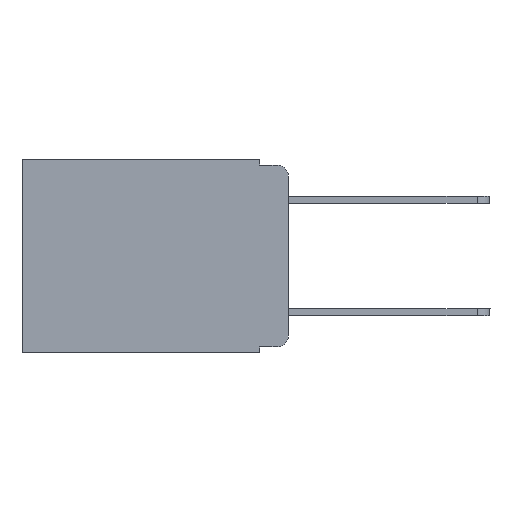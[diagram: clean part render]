
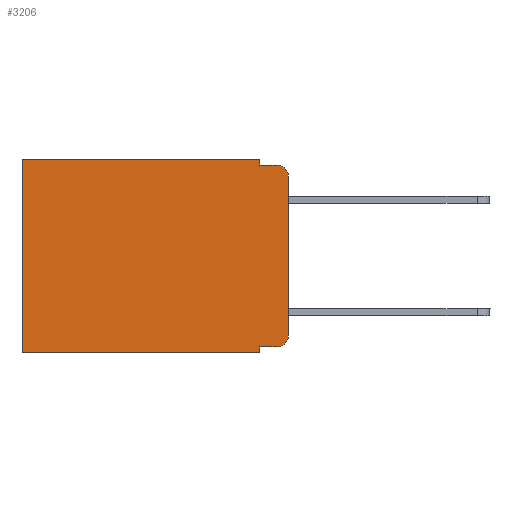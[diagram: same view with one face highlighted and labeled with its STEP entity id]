
A CAD part, left-side view. The second image highlights one B-rep face of the part: STEP entity #3206.
In plain terms, the highlighted planar face has unit normal (-1, 0, 0).
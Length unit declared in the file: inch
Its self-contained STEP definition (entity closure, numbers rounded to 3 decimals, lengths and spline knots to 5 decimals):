
#58 = DIRECTION ( 'NONE',  ( 1., 0., 0. ) ) ;
#177 = VERTEX_POINT ( 'NONE', #828 ) ;
#245 = VECTOR ( 'NONE', #8202, 39.37008 ) ;
#268 = CARTESIAN_POINT ( 'NONE',  ( 0.298, 0.051, -0.01 ) ) ;
#376 = VECTOR ( 'NONE', #6750, 39.37008 ) ;
#405 = VERTEX_POINT ( 'NONE', #2951 ) ;
#440 = EDGE_CURVE ( 'NONE', #177, #8833, #8044, .T. ) ;
#578 = ORIENTED_EDGE ( 'NONE', *, *, #5057, .T. ) ;
#694 = LINE ( 'NONE', #5782, #376 ) ;
#828 = CARTESIAN_POINT ( 'NONE',  ( 0.298, 0., -0.03 ) ) ;
#848 = AXIS2_PLACEMENT_3D ( 'NONE', #11522, #58, #8780 ) ;
#969 = EDGE_CURVE ( 'NONE', #11356, #11102, #1796, .T. ) ;
#1098 = CARTESIAN_POINT ( 'NONE',  ( 0.298, 0.473, 0. ) ) ;
#1139 = CARTESIAN_POINT ( 'NONE',  ( 0.298, 0., 0. ) ) ;
#1166 = DIRECTION ( 'NONE',  ( 0., -1., 0. ) ) ;
#1343 = VECTOR ( 'NONE', #5921, 39.37008 ) ;
#1364 = CARTESIAN_POINT ( 'NONE',  ( 0.298, 0.051, 0. ) ) ;
#1660 = EDGE_CURVE ( 'NONE', #2913, #10667, #4234, .T. ) ;
#1796 = LINE ( 'NONE', #1139, #1343 ) ;
#2114 = ORIENTED_EDGE ( 'NONE', *, *, #2936, .F. ) ;
#2369 = ORIENTED_EDGE ( 'NONE', *, *, #4551, .F. ) ;
#2622 = LINE ( 'NONE', #268, #12296 ) ;
#2631 = VERTEX_POINT ( 'NONE', #12217 ) ;
#2913 = VERTEX_POINT ( 'NONE', #6531 ) ;
#2936 = EDGE_CURVE ( 'NONE', #6580, #405, #11005, .T. ) ;
#2951 = CARTESIAN_POINT ( 'NONE',  ( 0.298, 0.473, -0.343 ) ) ;
#2954 = ORIENTED_EDGE ( 'NONE', *, *, #4802, .F. ) ;
#3108 = ORIENTED_EDGE ( 'NONE', *, *, #440, .T. ) ;
#3206 = ADVANCED_FACE ( 'NONE', ( #6634 ), #10573, .F. ) ;
#3431 = DIRECTION ( 'NONE',  ( 0., -1., 0. ) ) ;
#3469 = CARTESIAN_POINT ( 'NONE',  ( 0.298, 0., -0.343 ) ) ;
#3478 = CARTESIAN_POINT ( 'NONE',  ( 0.298, 0.02, -0.333 ) ) ;
#3560 = CARTESIAN_POINT ( 'NONE',  ( 0.298, 0.051, -0.333 ) ) ;
#3712 = EDGE_CURVE ( 'NONE', #11356, #5289, #694, .T. ) ;
#3851 = CARTESIAN_POINT ( 'NONE',  ( 0.298, 0.02, -0.313 ) ) ;
#4076 = ORIENTED_EDGE ( 'NONE', *, *, #969, .T. ) ;
#4234 = LINE ( 'NONE', #3560, #6826 ) ;
#4291 = DIRECTION ( 'NONE',  ( 0., 0., -1. ) ) ;
#4551 = EDGE_CURVE ( 'NONE', #177, #2631, #7924, .T. ) ;
#4648 = CIRCLE ( 'NONE', #8745, 0.02 ) ;
#4802 = EDGE_CURVE ( 'NONE', #5289, #8833, #2622, .T. ) ;
#5057 = EDGE_CURVE ( 'NONE', #11102, #405, #11379, .T. ) ;
#5289 = VERTEX_POINT ( 'NONE', #10189 ) ;
#5382 = DIRECTION ( 'NONE',  ( -1., 0., 0. ) ) ;
#5421 = CARTESIAN_POINT ( 'NONE',  ( 0.298, 0.02, -0.03 ) ) ;
#5782 = CARTESIAN_POINT ( 'NONE',  ( 0.298, 0.051, 0. ) ) ;
#5921 = DIRECTION ( 'NONE',  ( 0., 1., 0. ) ) ;
#6219 = CARTESIAN_POINT ( 'NONE',  ( 0.298, 0., 0. ) ) ;
#6531 = CARTESIAN_POINT ( 'NONE',  ( 0.298, 0.051, -0.333 ) ) ;
#6580 = VERTEX_POINT ( 'NONE', #11463 ) ;
#6634 = FACE_OUTER_BOUND ( 'NONE', #9726, .T. ) ;
#6750 = DIRECTION ( 'NONE',  ( 0., 0., -1. ) ) ;
#6792 = DIRECTION ( 'NONE',  ( 0., 0., -1. ) ) ;
#6826 = VECTOR ( 'NONE', #3431, 39.37008 ) ;
#7299 = CARTESIAN_POINT ( 'NONE',  ( 0.298, 0.02, -0.01 ) ) ;
#7401 = VECTOR ( 'NONE', #10286, 39.37008 ) ;
#7889 = DIRECTION ( 'NONE',  ( 0., 0., -1. ) ) ;
#7907 = ORIENTED_EDGE ( 'NONE', *, *, #1660, .T. ) ;
#7924 = LINE ( 'NONE', #6219, #11247 ) ;
#8044 = CIRCLE ( 'NONE', #9591, 0.02 ) ;
#8189 = DIRECTION ( 'NONE',  ( 0., 0., -1. ) ) ;
#8202 = DIRECTION ( 'NONE',  ( 0., 0., -1. ) ) ;
#8480 = CARTESIAN_POINT ( 'NONE',  ( 0.298, 0.473, 0. ) ) ;
#8745 = AXIS2_PLACEMENT_3D ( 'NONE', #3851, #10621, #6792 ) ;
#8780 = DIRECTION ( 'NONE',  ( 0., 0., -1. ) ) ;
#8833 = VERTEX_POINT ( 'NONE', #7299 ) ;
#8891 = LINE ( 'NONE', #1364, #245 ) ;
#8972 = EDGE_CURVE ( 'NONE', #10667, #2631, #4648, .T. ) ;
#9210 = ORIENTED_EDGE ( 'NONE', *, *, #11551, .F. ) ;
#9591 = AXIS2_PLACEMENT_3D ( 'NONE', #5421, #5382, #8189 ) ;
#9726 = EDGE_LOOP ( 'NONE', ( #2369, #3108, #2954, #12173, #4076, #578, #2114, #9210, #7907, #11196 ) ) ;
#10189 = CARTESIAN_POINT ( 'NONE',  ( 0.298, 0.051, -0.01 ) ) ;
#10286 = DIRECTION ( 'NONE',  ( 0., 1., 0. ) ) ;
#10573 = PLANE ( 'NONE',  #848 ) ;
#10621 = DIRECTION ( 'NONE',  ( -1., 0., 0. ) ) ;
#10667 = VERTEX_POINT ( 'NONE', #3478 ) ;
#11005 = LINE ( 'NONE', #3469, #7401 ) ;
#11102 = VERTEX_POINT ( 'NONE', #8480 ) ;
#11196 = ORIENTED_EDGE ( 'NONE', *, *, #8972, .T. ) ;
#11233 = VECTOR ( 'NONE', #7889, 39.37008 ) ;
#11247 = VECTOR ( 'NONE', #4291, 39.37008 ) ;
#11356 = VERTEX_POINT ( 'NONE', #11758 ) ;
#11379 = LINE ( 'NONE', #1098, #11233 ) ;
#11463 = CARTESIAN_POINT ( 'NONE',  ( 0.298, 0.051, -0.343 ) ) ;
#11522 = CARTESIAN_POINT ( 'NONE',  ( 0.298, 0., 0. ) ) ;
#11551 = EDGE_CURVE ( 'NONE', #2913, #6580, #8891, .T. ) ;
#11758 = CARTESIAN_POINT ( 'NONE',  ( 0.298, 0.051, 0. ) ) ;
#12173 = ORIENTED_EDGE ( 'NONE', *, *, #3712, .F. ) ;
#12217 = CARTESIAN_POINT ( 'NONE',  ( 0.298, 0., -0.313 ) ) ;
#12296 = VECTOR ( 'NONE', #1166, 39.37008 ) ;
